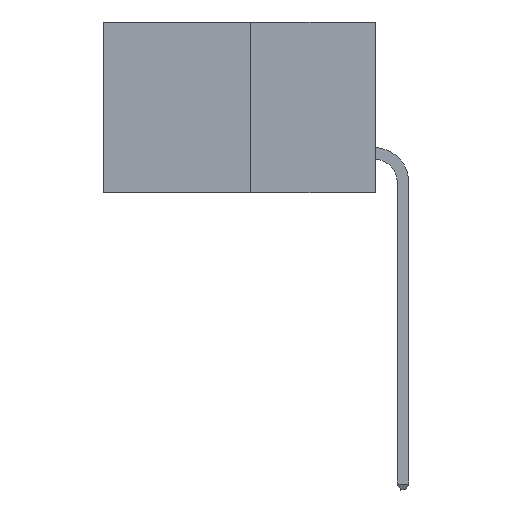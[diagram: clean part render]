
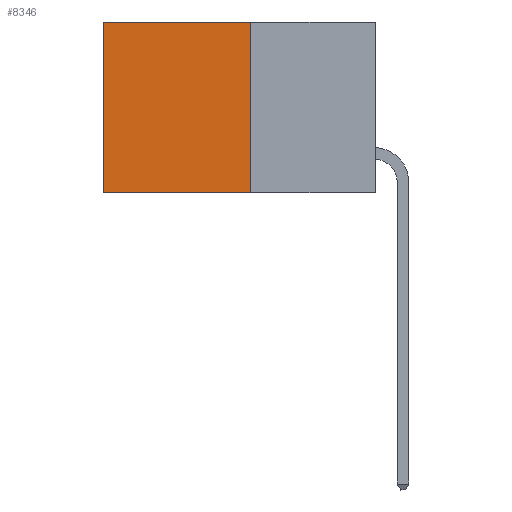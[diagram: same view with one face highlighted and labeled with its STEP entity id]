
A CAD part, left-side view. The second image highlights one B-rep face of the part: STEP entity #8346.
In plain terms, the highlighted planar face has unit normal (-1, 0, 0).
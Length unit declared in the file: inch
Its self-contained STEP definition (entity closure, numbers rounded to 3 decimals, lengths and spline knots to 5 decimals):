
#664 = EDGE_LOOP ( 'NONE', ( #13614, #11756, #14013, #18588 ) ) ;
#1052 = CARTESIAN_POINT ( 'NONE',  ( 0.277, 0.27, 0. ) ) ;
#1496 = VERTEX_POINT ( 'NONE', #5064 ) ;
#1582 = DIRECTION ( 'NONE',  ( 0., 0., -1. ) ) ;
#1735 = EDGE_CURVE ( 'NONE', #16763, #1818, #7072, .T. ) ;
#1818 = VERTEX_POINT ( 'NONE', #3161 ) ;
#1903 = CARTESIAN_POINT ( 'NONE',  ( 0.277, 0.27, 0. ) ) ;
#3161 = CARTESIAN_POINT ( 'NONE',  ( 0.277, 0.59, -0.37 ) ) ;
#3738 = CARTESIAN_POINT ( 'NONE',  ( 0.277, 0.27, -0.37 ) ) ;
#5064 = CARTESIAN_POINT ( 'NONE',  ( 0.277, 0.27, -0.37 ) ) ;
#6188 = VERTEX_POINT ( 'NONE', #1052 ) ;
#7072 = LINE ( 'NONE', #16010, #19952 ) ;
#7290 = DIRECTION ( 'NONE',  ( 0., 0., -1. ) ) ;
#8346 = ADVANCED_FACE ( 'NONE', ( #9150 ), #20346, .F. ) ;
#8687 = DIRECTION ( 'NONE',  ( 0., 0., -1. ) ) ;
#9113 = VECTOR ( 'NONE', #8687, 39.37008 ) ;
#9150 = FACE_OUTER_BOUND ( 'NONE', #664, .T. ) ;
#10454 = CARTESIAN_POINT ( 'NONE',  ( 0.277, 0.59, 0. ) ) ;
#11136 = DIRECTION ( 'NONE',  ( 1., 0., 0. ) ) ;
#11260 = LINE ( 'NONE', #3738, #18535 ) ;
#11756 = ORIENTED_EDGE ( 'NONE', *, *, #12815, .F. ) ;
#12325 = LINE ( 'NONE', #16480, #9113 ) ;
#12815 = EDGE_CURVE ( 'NONE', #1496, #1818, #11260, .T. ) ;
#13614 = ORIENTED_EDGE ( 'NONE', *, *, #1735, .T. ) ;
#14013 = ORIENTED_EDGE ( 'NONE', *, *, #18814, .F. ) ;
#14585 = AXIS2_PLACEMENT_3D ( 'NONE', #15764, #11136, #1582 ) ;
#15736 = VECTOR ( 'NONE', #16148, 39.37008 ) ;
#15764 = CARTESIAN_POINT ( 'NONE',  ( 0.277, 0.27, -0.37 ) ) ;
#16010 = CARTESIAN_POINT ( 'NONE',  ( 0.277, 0.59, -0.37 ) ) ;
#16148 = DIRECTION ( 'NONE',  ( 0., 1., 0. ) ) ;
#16233 = LINE ( 'NONE', #1903, #15736 ) ;
#16373 = DIRECTION ( 'NONE',  ( 0., 1., 0. ) ) ;
#16480 = CARTESIAN_POINT ( 'NONE',  ( 0.277, 0.27, -0.37 ) ) ;
#16763 = VERTEX_POINT ( 'NONE', #10454 ) ;
#18535 = VECTOR ( 'NONE', #16373, 39.37008 ) ;
#18588 = ORIENTED_EDGE ( 'NONE', *, *, #18671, .T. ) ;
#18671 = EDGE_CURVE ( 'NONE', #6188, #16763, #16233, .T. ) ;
#18814 = EDGE_CURVE ( 'NONE', #6188, #1496, #12325, .T. ) ;
#19952 = VECTOR ( 'NONE', #7290, 39.37008 ) ;
#20346 = PLANE ( 'NONE',  #14585 ) ;
